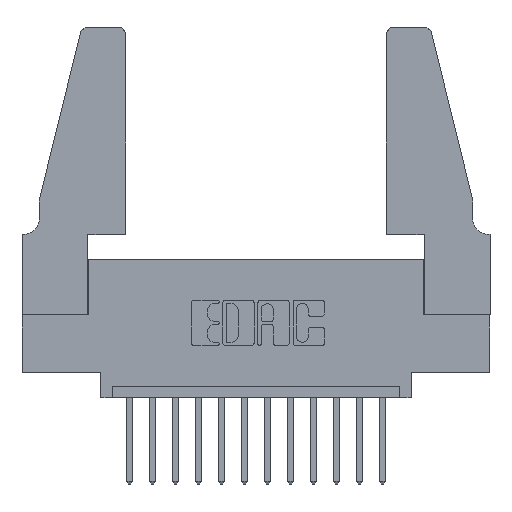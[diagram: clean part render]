
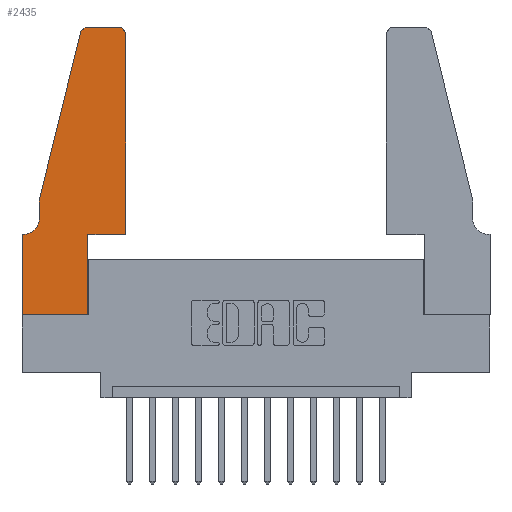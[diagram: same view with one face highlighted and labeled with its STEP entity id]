
A CAD part, top view. The second image highlights one B-rep face of the part: STEP entity #2435.
In plain terms, the highlighted planar face has unit normal (0, 0, 1).
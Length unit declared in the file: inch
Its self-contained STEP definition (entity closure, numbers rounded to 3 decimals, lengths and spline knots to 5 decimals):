
#204 = LINE ( 'NONE', #7548, #2635 ) ;
#262 = DIRECTION ( 'NONE',  ( -1., 0., 0. ) ) ;
#386 = VECTOR ( 'NONE', #4458, 39.37008 ) ;
#802 = DIRECTION ( 'NONE',  ( 0., 0., 1. ) ) ;
#850 = CARTESIAN_POINT ( 'NONE',  ( 0.25487, 1.22718, 0.37 ) ) ;
#1380 = CARTESIAN_POINT ( 'NONE',  ( 0.284, 1.25, 0.37 ) ) ;
#1593 = CARTESIAN_POINT ( 'NONE',  ( 0., 0., 0.37 ) ) ;
#1616 = CARTESIAN_POINT ( 'NONE',  ( 0.0055, 0.42, 0.37 ) ) ;
#2020 = EDGE_CURVE ( 'NONE', #14887, #11554, #10312, .T. ) ;
#2044 = VERTEX_POINT ( 'NONE', #11759 ) ;
#2144 = CARTESIAN_POINT ( 'NONE',  ( 0.0755, 0.5, 0.37 ) ) ;
#2146 = VERTEX_POINT ( 'NONE', #1380 ) ;
#2303 = EDGE_LOOP ( 'NONE', ( #13640, #11655, #6741, #5623, #10317, #8199, #3887, #15262, #6342, #10285, #7055, #13198 ) ) ;
#2435 = ADVANCED_FACE ( 'NONE', ( #11093 ), #9213, .T. ) ;
#2635 = VECTOR ( 'NONE', #7442, 39.37008 ) ;
#2681 = CARTESIAN_POINT ( 'NONE',  ( 0.284, 1.22, 0.37 ) ) ;
#2832 = CARTESIAN_POINT ( 'NONE',  ( 0., 0., 0.37 ) ) ;
#2962 = VECTOR ( 'NONE', #12326, 39.37008 ) ;
#3368 = CARTESIAN_POINT ( 'NONE',  ( 0.0755, 0.5, 0.37 ) ) ;
#3470 = DIRECTION ( 'NONE',  ( 0., -1., 0. ) ) ;
#3594 = AXIS2_PLACEMENT_3D ( 'NONE', #2681, #10905, #11047 ) ;
#3694 = VECTOR ( 'NONE', #13963, 39.37008 ) ;
#3705 = EDGE_CURVE ( 'NONE', #2044, #4652, #8249, .T. ) ;
#3887 = ORIENTED_EDGE ( 'NONE', *, *, #6482, .T. ) ;
#3963 = DIRECTION ( 'NONE',  ( 0., 0., -1. ) ) ;
#4181 = VECTOR ( 'NONE', #5840, 39.37008 ) ;
#4194 = VERTEX_POINT ( 'NONE', #6493 ) ;
#4380 = DIRECTION ( 'NONE',  ( 0., 0., 1. ) ) ;
#4458 = DIRECTION ( 'NONE',  ( 0., 1., 0. ) ) ;
#4552 = EDGE_CURVE ( 'NONE', #4194, #2146, #8536, .T. ) ;
#4652 = VERTEX_POINT ( 'NONE', #13098 ) ;
#4996 = VERTEX_POINT ( 'NONE', #5214 ) ;
#5054 = AXIS2_PLACEMENT_3D ( 'NONE', #11468, #802, #9142 ) ;
#5090 = EDGE_CURVE ( 'NONE', #4652, #11411, #204, .T. ) ;
#5214 = CARTESIAN_POINT ( 'NONE',  ( 0.0055, 0.35, 0.37 ) ) ;
#5391 = EDGE_CURVE ( 'NONE', #11770, #2044, #14886, .T. ) ;
#5551 = EDGE_CURVE ( 'NONE', #2146, #12093, #8767, .T. ) ;
#5623 = ORIENTED_EDGE ( 'NONE', *, *, #2020, .T. ) ;
#5840 = DIRECTION ( 'NONE',  ( 1., 0., 0. ) ) ;
#6100 = VECTOR ( 'NONE', #12265, 39.37008 ) ;
#6342 = ORIENTED_EDGE ( 'NONE', *, *, #5391, .T. ) ;
#6482 = EDGE_CURVE ( 'NONE', #10835, #7946, #9832, .T. ) ;
#6486 = AXIS2_PLACEMENT_3D ( 'NONE', #1616, #3963, #262 ) ;
#6493 = CARTESIAN_POINT ( 'NONE',  ( 0.4205, 1.25, 0.37 ) ) ;
#6636 = EDGE_CURVE ( 'NONE', #4996, #10835, #13535, .T. ) ;
#6741 = ORIENTED_EDGE ( 'NONE', *, *, #10716, .T. ) ;
#6783 = DIRECTION ( 'NONE',  ( 1., 0., 0. ) ) ;
#7055 = ORIENTED_EDGE ( 'NONE', *, *, #5090, .T. ) ;
#7442 = DIRECTION ( 'NONE',  ( 0., 1., 0. ) ) ;
#7548 = CARTESIAN_POINT ( 'NONE',  ( 0.4505, 0.35, 0.37 ) ) ;
#7701 = CARTESIAN_POINT ( 'NONE',  ( 0., 0., 0.37 ) ) ;
#7721 = EDGE_CURVE ( 'NONE', #11554, #4996, #10922, .T. ) ;
#7930 = CIRCLE ( 'NONE', #5054, 0.03 ) ;
#7946 = VERTEX_POINT ( 'NONE', #2832 ) ;
#8092 = CARTESIAN_POINT ( 'NONE',  ( 0.0755, 0.35, 0.37 ) ) ;
#8199 = ORIENTED_EDGE ( 'NONE', *, *, #6636, .T. ) ;
#8249 = LINE ( 'NONE', #12913, #4181 ) ;
#8536 = LINE ( 'NONE', #10670, #6100 ) ;
#8767 = CIRCLE ( 'NONE', #3594, 0.03 ) ;
#9142 = DIRECTION ( 'NONE',  ( 1., 0., 0. ) ) ;
#9213 = PLANE ( 'NONE',  #9561 ) ;
#9527 = EDGE_CURVE ( 'NONE', #7946, #11770, #10061, .T. ) ;
#9561 = AXIS2_PLACEMENT_3D ( 'NONE', #13923, #4380, #6783 ) ;
#9768 = VECTOR ( 'NONE', #3470, 39.37008 ) ;
#9832 = LINE ( 'NONE', #1593, #2962 ) ;
#9957 = DIRECTION ( 'NONE',  ( 1., 0., 0. ) ) ;
#9982 = CARTESIAN_POINT ( 'NONE',  ( 0.4505, 1.22, 0.37 ) ) ;
#10061 = LINE ( 'NONE', #7701, #15269 ) ;
#10285 = ORIENTED_EDGE ( 'NONE', *, *, #3705, .T. ) ;
#10312 = LINE ( 'NONE', #3368, #9768 ) ;
#10317 = ORIENTED_EDGE ( 'NONE', *, *, #7721, .T. ) ;
#10670 = CARTESIAN_POINT ( 'NONE',  ( 0.2605, 1.25, 0.37 ) ) ;
#10716 = EDGE_CURVE ( 'NONE', #12093, #14887, #15064, .T. ) ;
#10835 = VERTEX_POINT ( 'NONE', #11469 ) ;
#10905 = DIRECTION ( 'NONE',  ( 0., 0., 1. ) ) ;
#10922 = CIRCLE ( 'NONE', #6486, 0.07 ) ;
#11047 = DIRECTION ( 'NONE',  ( 1., 0., 0. ) ) ;
#11093 = FACE_OUTER_BOUND ( 'NONE', #2303, .T. ) ;
#11411 = VERTEX_POINT ( 'NONE', #9982 ) ;
#11468 = CARTESIAN_POINT ( 'NONE',  ( 0.4205, 1.22, 0.37 ) ) ;
#11469 = CARTESIAN_POINT ( 'NONE',  ( 0., 0.35, 0.37 ) ) ;
#11553 = CARTESIAN_POINT ( 'NONE',  ( 0.0755, 0.42, 0.37 ) ) ;
#11554 = VERTEX_POINT ( 'NONE', #11553 ) ;
#11655 = ORIENTED_EDGE ( 'NONE', *, *, #5551, .T. ) ;
#11671 = DIRECTION ( 'NONE',  ( -0.239, -0.971, 0. ) ) ;
#11759 = CARTESIAN_POINT ( 'NONE',  ( 0.2865, 0.35, 0.37 ) ) ;
#11770 = VERTEX_POINT ( 'NONE', #15288 ) ;
#12093 = VERTEX_POINT ( 'NONE', #850 ) ;
#12186 = EDGE_CURVE ( 'NONE', #11411, #4194, #7930, .T. ) ;
#12265 = DIRECTION ( 'NONE',  ( -1., 0., 0. ) ) ;
#12326 = DIRECTION ( 'NONE',  ( 0., -1., 0. ) ) ;
#12913 = CARTESIAN_POINT ( 'NONE',  ( 0.4505, 0.35, 0.37 ) ) ;
#13098 = CARTESIAN_POINT ( 'NONE',  ( 0.4505, 0.35, 0.37 ) ) ;
#13198 = ORIENTED_EDGE ( 'NONE', *, *, #12186, .T. ) ;
#13331 = CARTESIAN_POINT ( 'NONE',  ( 0.0755, 0.5, 0.37 ) ) ;
#13535 = LINE ( 'NONE', #8092, #3694 ) ;
#13640 = ORIENTED_EDGE ( 'NONE', *, *, #4552, .T. ) ;
#13906 = CARTESIAN_POINT ( 'NONE',  ( 0.2865, 0.35, 0.37 ) ) ;
#13923 = CARTESIAN_POINT ( 'NONE',  ( 0., 0.35, 0.37 ) ) ;
#13963 = DIRECTION ( 'NONE',  ( -1., 0., 0. ) ) ;
#14319 = VECTOR ( 'NONE', #11671, 39.37008 ) ;
#14886 = LINE ( 'NONE', #13906, #386 ) ;
#14887 = VERTEX_POINT ( 'NONE', #13331 ) ;
#15064 = LINE ( 'NONE', #2144, #14319 ) ;
#15262 = ORIENTED_EDGE ( 'NONE', *, *, #9527, .T. ) ;
#15269 = VECTOR ( 'NONE', #9957, 39.37008 ) ;
#15288 = CARTESIAN_POINT ( 'NONE',  ( 0.2865, 0., 0.37 ) ) ;
